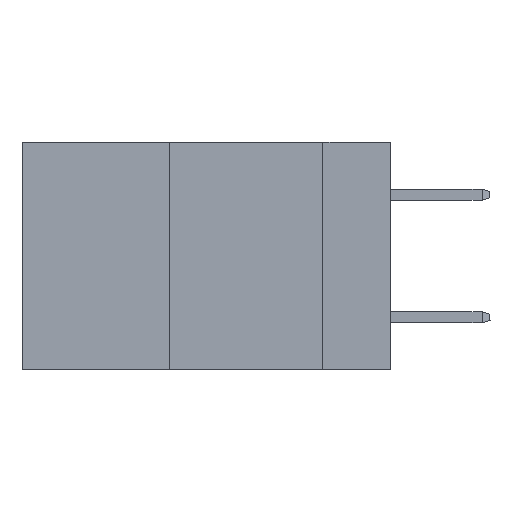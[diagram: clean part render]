
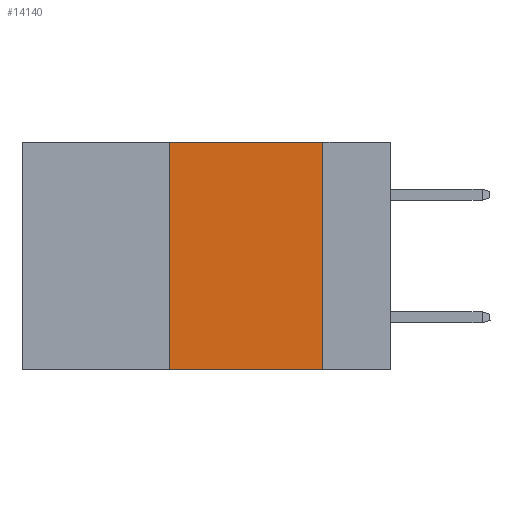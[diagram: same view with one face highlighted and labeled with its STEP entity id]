
A CAD part, left-side view. The second image highlights one B-rep face of the part: STEP entity #14140.
In plain terms, the highlighted planar face has unit normal (-1, 0, 0).
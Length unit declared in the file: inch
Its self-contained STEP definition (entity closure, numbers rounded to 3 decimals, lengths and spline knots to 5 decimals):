
#70 = ORIENTED_EDGE ( 'NONE', *, *, #1236, .F. ) ;
#266 = CARTESIAN_POINT ( 'NONE',  ( 0., 0.11, -0.37 ) ) ;
#1236 = EDGE_CURVE ( 'NONE', #9742, #13419, #5441, .T. ) ;
#2485 = VECTOR ( 'NONE', #3988, 39.37008 ) ;
#3126 = VERTEX_POINT ( 'NONE', #8098 ) ;
#3988 = DIRECTION ( 'NONE',  ( 0., -1., 0. ) ) ;
#4165 = EDGE_CURVE ( 'NONE', #12453, #3126, #11198, .T. ) ;
#4432 = FACE_OUTER_BOUND ( 'NONE', #14366, .T. ) ;
#5441 = LINE ( 'NONE', #9780, #12869 ) ;
#5826 = LINE ( 'NONE', #7401, #2485 ) ;
#6095 = DIRECTION ( 'NONE',  ( 0., 0., -1. ) ) ;
#6607 = EDGE_CURVE ( 'NONE', #12453, #13419, #16202, .T. ) ;
#6928 = CARTESIAN_POINT ( 'NONE',  ( 0., 0.11, 0. ) ) ;
#7401 = CARTESIAN_POINT ( 'NONE',  ( 0., 0.6, 0. ) ) ;
#8098 = CARTESIAN_POINT ( 'NONE',  ( 0., 0.36, 0. ) ) ;
#8959 = CARTESIAN_POINT ( 'NONE',  ( 0., 0.6, 0. ) ) ;
#9336 = CARTESIAN_POINT ( 'NONE',  ( 0., 0.6, -0.37 ) ) ;
#9742 = VERTEX_POINT ( 'NONE', #6928 ) ;
#9780 = CARTESIAN_POINT ( 'NONE',  ( 0., 0.11, 0. ) ) ;
#9953 = ORIENTED_EDGE ( 'NONE', *, *, #6607, .T. ) ;
#10215 = VECTOR ( 'NONE', #11696, 39.37008 ) ;
#10723 = DIRECTION ( 'NONE',  ( 0., -1., 0. ) ) ;
#11198 = LINE ( 'NONE', #14203, #10215 ) ;
#11643 = EDGE_CURVE ( 'NONE', #3126, #9742, #5826, .T. ) ;
#11696 = DIRECTION ( 'NONE',  ( 0., 0., 1. ) ) ;
#11910 = AXIS2_PLACEMENT_3D ( 'NONE', #8959, #15268, #6095 ) ;
#12453 = VERTEX_POINT ( 'NONE', #15405 ) ;
#12484 = ORIENTED_EDGE ( 'NONE', *, *, #4165, .F. ) ;
#12869 = VECTOR ( 'NONE', #13587, 39.37008 ) ;
#13419 = VERTEX_POINT ( 'NONE', #266 ) ;
#13587 = DIRECTION ( 'NONE',  ( 0., 0., -1. ) ) ;
#14140 = ADVANCED_FACE ( 'NONE', ( #4432 ), #14619, .F. ) ;
#14203 = CARTESIAN_POINT ( 'NONE',  ( 0., 0.36, 0. ) ) ;
#14366 = EDGE_LOOP ( 'NONE', ( #70, #14755, #12484, #9953 ) ) ;
#14435 = VECTOR ( 'NONE', #10723, 39.37008 ) ;
#14619 = PLANE ( 'NONE',  #11910 ) ;
#14755 = ORIENTED_EDGE ( 'NONE', *, *, #11643, .F. ) ;
#15268 = DIRECTION ( 'NONE',  ( 1., 0., 0. ) ) ;
#15405 = CARTESIAN_POINT ( 'NONE',  ( 0., 0.36, -0.37 ) ) ;
#16202 = LINE ( 'NONE', #9336, #14435 ) ;
